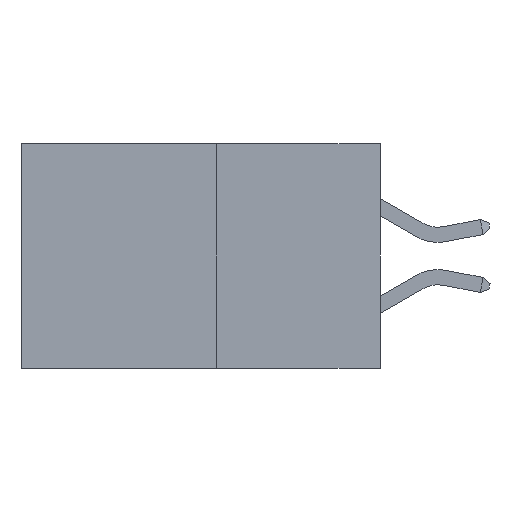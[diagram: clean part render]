
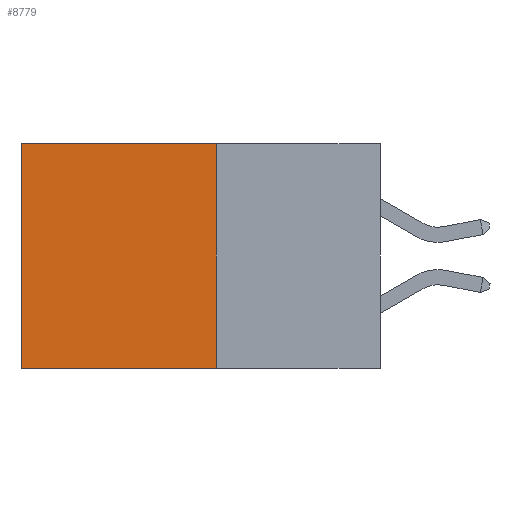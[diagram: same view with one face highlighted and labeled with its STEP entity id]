
A CAD part, left-side view. The second image highlights one B-rep face of the part: STEP entity #8779.
In plain terms, the highlighted planar face has unit normal (-1, 0, 0).
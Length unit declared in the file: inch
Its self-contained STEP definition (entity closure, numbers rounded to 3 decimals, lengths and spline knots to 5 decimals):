
#5 = VERTEX_POINT ( 'NONE', #4663 ) ;
#531 = ORIENTED_EDGE ( 'NONE', *, *, #2422, .T. ) ;
#869 = VECTOR ( 'NONE', #9057, 39.37008 ) ;
#992 = PLANE ( 'NONE',  #1326 ) ;
#1326 = AXIS2_PLACEMENT_3D ( 'NONE', #6577, #7348, #2604 ) ;
#1389 = ORIENTED_EDGE ( 'NONE', *, *, #5847, .T. ) ;
#1466 = VERTEX_POINT ( 'NONE', #6774 ) ;
#1592 = LINE ( 'NONE', #6931, #7900 ) ;
#1687 = CARTESIAN_POINT ( 'NONE',  ( 0.277, 0.27, -0.37 ) ) ;
#1878 = CARTESIAN_POINT ( 'NONE',  ( 0.277, 0.59, 0. ) ) ;
#2422 = EDGE_CURVE ( 'NONE', #4209, #5, #1592, .T. ) ;
#2604 = DIRECTION ( 'NONE',  ( 0., 0., -1. ) ) ;
#2785 = DIRECTION ( 'NONE',  ( 0., 0., -1. ) ) ;
#3055 = VECTOR ( 'NONE', #5364, 39.37008 ) ;
#3300 = LINE ( 'NONE', #5473, #3055 ) ;
#3383 = EDGE_LOOP ( 'NONE', ( #531, #7231, #7467, #1389 ) ) ;
#3480 = LINE ( 'NONE', #8299, #7465 ) ;
#4209 = VERTEX_POINT ( 'NONE', #1878 ) ;
#4663 = CARTESIAN_POINT ( 'NONE',  ( 0.277, 0.59, -0.37 ) ) ;
#5140 = LINE ( 'NONE', #9073, #869 ) ;
#5364 = DIRECTION ( 'NONE',  ( 0., 1., 0. ) ) ;
#5473 = CARTESIAN_POINT ( 'NONE',  ( 0.277, 0.27, -0.37 ) ) ;
#5591 = VERTEX_POINT ( 'NONE', #1687 ) ;
#5847 = EDGE_CURVE ( 'NONE', #1466, #4209, #5140, .T. ) ;
#6577 = CARTESIAN_POINT ( 'NONE',  ( 0.277, 0.27, -0.37 ) ) ;
#6774 = CARTESIAN_POINT ( 'NONE',  ( 0.277, 0.27, 0. ) ) ;
#6931 = CARTESIAN_POINT ( 'NONE',  ( 0.277, 0.59, -0.37 ) ) ;
#7231 = ORIENTED_EDGE ( 'NONE', *, *, #7795, .F. ) ;
#7348 = DIRECTION ( 'NONE',  ( 1., 0., 0. ) ) ;
#7465 = VECTOR ( 'NONE', #2785, 39.37008 ) ;
#7467 = ORIENTED_EDGE ( 'NONE', *, *, #9589, .F. ) ;
#7795 = EDGE_CURVE ( 'NONE', #5591, #5, #3300, .T. ) ;
#7900 = VECTOR ( 'NONE', #10017, 39.37008 ) ;
#8299 = CARTESIAN_POINT ( 'NONE',  ( 0.277, 0.27, -0.37 ) ) ;
#8344 = FACE_OUTER_BOUND ( 'NONE', #3383, .T. ) ;
#8779 = ADVANCED_FACE ( 'NONE', ( #8344 ), #992, .F. ) ;
#9057 = DIRECTION ( 'NONE',  ( 0., 1., 0. ) ) ;
#9073 = CARTESIAN_POINT ( 'NONE',  ( 0.277, 0.27, 0. ) ) ;
#9589 = EDGE_CURVE ( 'NONE', #1466, #5591, #3480, .T. ) ;
#10017 = DIRECTION ( 'NONE',  ( 0., 0., -1. ) ) ;
